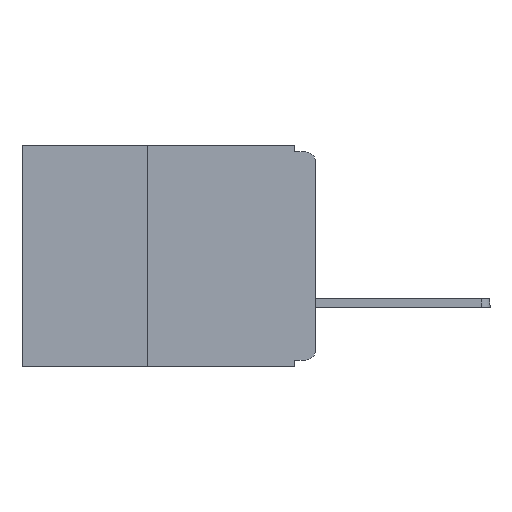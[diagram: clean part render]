
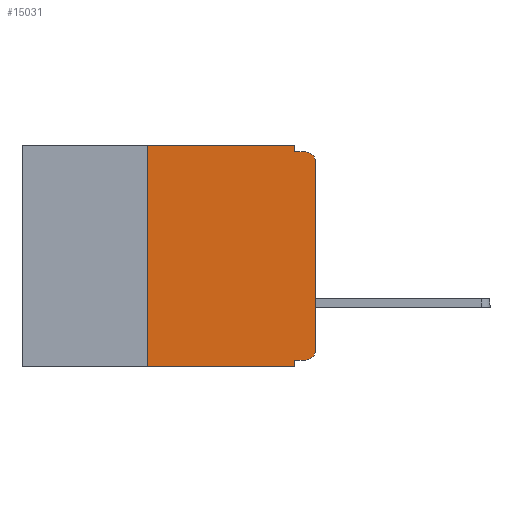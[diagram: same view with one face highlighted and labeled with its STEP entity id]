
A CAD part, left-side view. The second image highlights one B-rep face of the part: STEP entity #15031.
In plain terms, the highlighted planar face has unit normal (-1, 0, 0).
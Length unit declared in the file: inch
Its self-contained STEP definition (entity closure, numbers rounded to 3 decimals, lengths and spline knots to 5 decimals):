
#36 = FACE_OUTER_BOUND ( 'NONE', #22014, .T. ) ;
#325 = EDGE_CURVE ( 'NONE', #5079, #30346, #10696, .T. ) ;
#528 = VERTEX_POINT ( 'NONE', #1846 ) ;
#604 = LINE ( 'NONE', #11345, #18963 ) ;
#650 = VECTOR ( 'NONE', #10641, 39.37008 ) ;
#1252 = DIRECTION ( 'NONE',  ( 0., 1., 0. ) ) ;
#1643 = CARTESIAN_POINT ( 'NONE',  ( 0., 0.015, -0.01 ) ) ;
#1846 = CARTESIAN_POINT ( 'NONE',  ( 0., 0.25, 0. ) ) ;
#2045 = EDGE_CURVE ( 'NONE', #3854, #26957, #28303, .T. ) ;
#2236 = ORIENTED_EDGE ( 'NONE', *, *, #23727, .F. ) ;
#2573 = DIRECTION ( 'NONE',  ( 0., -1., 0. ) ) ;
#2859 = VERTEX_POINT ( 'NONE', #24606 ) ;
#3403 = DIRECTION ( 'NONE',  ( 0., 0., -1. ) ) ;
#3755 = CIRCLE ( 'NONE', #9230, 0.015 ) ;
#3854 = VERTEX_POINT ( 'NONE', #4088 ) ;
#4088 = CARTESIAN_POINT ( 'NONE',  ( 0., 0.031, -0.32 ) ) ;
#4445 = CARTESIAN_POINT ( 'NONE',  ( 0., 0., -0.305 ) ) ;
#4641 = EDGE_CURVE ( 'NONE', #6020, #7470, #3755, .T. ) ;
#4843 = ORIENTED_EDGE ( 'NONE', *, *, #24365, .T. ) ;
#5079 = VERTEX_POINT ( 'NONE', #19628 ) ;
#5269 = DIRECTION ( 'NONE',  ( 0., 0., -1. ) ) ;
#6014 = CARTESIAN_POINT ( 'NONE',  ( 0., 0., -0.32 ) ) ;
#6020 = VERTEX_POINT ( 'NONE', #22415 ) ;
#6317 = AXIS2_PLACEMENT_3D ( 'NONE', #28609, #7527, #3403 ) ;
#6527 = DIRECTION ( 'NONE',  ( 0., 0., -1. ) ) ;
#6744 = LINE ( 'NONE', #30148, #30242 ) ;
#6793 = EDGE_CURVE ( 'NONE', #30346, #6020, #604, .T. ) ;
#6850 = ORIENTED_EDGE ( 'NONE', *, *, #2045, .F. ) ;
#6895 = ORIENTED_EDGE ( 'NONE', *, *, #28866, .F. ) ;
#7099 = ORIENTED_EDGE ( 'NONE', *, *, #19360, .F. ) ;
#7438 = CARTESIAN_POINT ( 'NONE',  ( 0., 0., -0.01 ) ) ;
#7470 = VERTEX_POINT ( 'NONE', #1643 ) ;
#7527 = DIRECTION ( 'NONE',  ( -1., 0., 0. ) ) ;
#8133 = ORIENTED_EDGE ( 'NONE', *, *, #325, .T. ) ;
#8624 = VERTEX_POINT ( 'NONE', #21074 ) ;
#9168 = DIRECTION ( 'NONE',  ( 0., -1., 0. ) ) ;
#9230 = AXIS2_PLACEMENT_3D ( 'NONE', #9524, #9489, #9454 ) ;
#9275 = CARTESIAN_POINT ( 'NONE',  ( 0., 0.437, -0.33 ) ) ;
#9454 = DIRECTION ( 'NONE',  ( 0., 0., -1. ) ) ;
#9489 = DIRECTION ( 'NONE',  ( -1., 0., 0. ) ) ;
#9524 = CARTESIAN_POINT ( 'NONE',  ( 0., 0.015, -0.025 ) ) ;
#9588 = VECTOR ( 'NONE', #24987, 39.37008 ) ;
#9981 = VECTOR ( 'NONE', #5269, 39.37008 ) ;
#10022 = VECTOR ( 'NONE', #1252, 39.37008 ) ;
#10641 = DIRECTION ( 'NONE',  ( 0., 0., 1. ) ) ;
#10696 = CIRCLE ( 'NONE', #6317, 0.015 ) ;
#11120 = ORIENTED_EDGE ( 'NONE', *, *, #4641, .T. ) ;
#11145 = CARTESIAN_POINT ( 'NONE',  ( 0., 0.25, -0.33 ) ) ;
#11345 = CARTESIAN_POINT ( 'NONE',  ( 0., 0., 0. ) ) ;
#11412 = DIRECTION ( 'NONE',  ( 0., 0., 1. ) ) ;
#12376 = ORIENTED_EDGE ( 'NONE', *, *, #26127, .F. ) ;
#12987 = CARTESIAN_POINT ( 'NONE',  ( 0., 0.25, -0.33 ) ) ;
#13159 = VERTEX_POINT ( 'NONE', #11145 ) ;
#14365 = ORIENTED_EDGE ( 'NONE', *, *, #6793, .T. ) ;
#14513 = CARTESIAN_POINT ( 'NONE',  ( 0., 0.031, -0.33 ) ) ;
#14936 = CARTESIAN_POINT ( 'NONE',  ( 0., 0.031, 0. ) ) ;
#15031 = ADVANCED_FACE ( 'NONE', ( #36 ), #18398, .F. ) ;
#15406 = LINE ( 'NONE', #7438, #20916 ) ;
#16263 = DIRECTION ( 'NONE',  ( 0., -1., 0. ) ) ;
#16411 = EDGE_CURVE ( 'NONE', #2859, #7470, #15406, .T. ) ;
#18398 = PLANE ( 'NONE',  #25867 ) ;
#18963 = VECTOR ( 'NONE', #11412, 39.37008 ) ;
#19360 = EDGE_CURVE ( 'NONE', #5079, #3854, #29444, .T. ) ;
#19628 = CARTESIAN_POINT ( 'NONE',  ( 0., 0.015, -0.32 ) ) ;
#19741 = LINE ( 'NONE', #12987, #650 ) ;
#20071 = VECTOR ( 'NONE', #9168, 39.37008 ) ;
#20764 = DIRECTION ( 'NONE',  ( 1., 0., 0. ) ) ;
#20916 = VECTOR ( 'NONE', #2573, 39.37008 ) ;
#21074 = CARTESIAN_POINT ( 'NONE',  ( 0., 0.031, 0. ) ) ;
#21815 = LINE ( 'NONE', #14936, #9981 ) ;
#22014 = EDGE_LOOP ( 'NONE', ( #14365, #11120, #26286, #6895, #12376, #2236, #4843, #6850, #7099, #8133 ) ) ;
#22415 = CARTESIAN_POINT ( 'NONE',  ( 0., 0., -0.025 ) ) ;
#23727 = EDGE_CURVE ( 'NONE', #13159, #528, #19741, .T. ) ;
#24292 = CARTESIAN_POINT ( 'NONE',  ( 0., 0.031, -0.33 ) ) ;
#24365 = EDGE_CURVE ( 'NONE', #13159, #26957, #26292, .T. ) ;
#24606 = CARTESIAN_POINT ( 'NONE',  ( 0., 0.031, -0.01 ) ) ;
#24987 = DIRECTION ( 'NONE',  ( 0., 0., -1. ) ) ;
#25867 = AXIS2_PLACEMENT_3D ( 'NONE', #27665, #20764, #6527 ) ;
#26127 = EDGE_CURVE ( 'NONE', #528, #8624, #6744, .T. ) ;
#26286 = ORIENTED_EDGE ( 'NONE', *, *, #16411, .F. ) ;
#26292 = LINE ( 'NONE', #9275, #20071 ) ;
#26957 = VERTEX_POINT ( 'NONE', #14513 ) ;
#27665 = CARTESIAN_POINT ( 'NONE',  ( 0., 0.437, 0. ) ) ;
#28303 = LINE ( 'NONE', #24292, #9588 ) ;
#28609 = CARTESIAN_POINT ( 'NONE',  ( 0., 0.015, -0.305 ) ) ;
#28866 = EDGE_CURVE ( 'NONE', #8624, #2859, #21815, .T. ) ;
#29444 = LINE ( 'NONE', #6014, #10022 ) ;
#30148 = CARTESIAN_POINT ( 'NONE',  ( 0., 0.437, 0. ) ) ;
#30242 = VECTOR ( 'NONE', #16263, 39.37008 ) ;
#30346 = VERTEX_POINT ( 'NONE', #4445 ) ;
